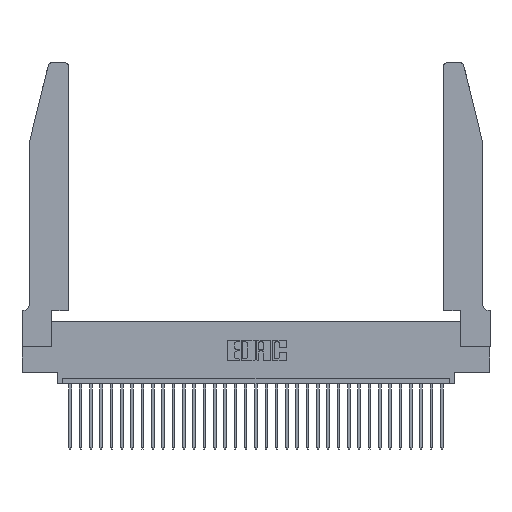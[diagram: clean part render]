
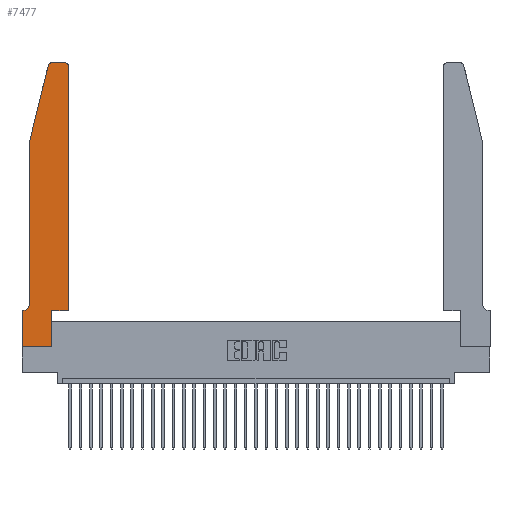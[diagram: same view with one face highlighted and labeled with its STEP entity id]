
A CAD part, top view. The second image highlights one B-rep face of the part: STEP entity #7477.
In plain terms, the highlighted planar face has unit normal (0, 0, 1).
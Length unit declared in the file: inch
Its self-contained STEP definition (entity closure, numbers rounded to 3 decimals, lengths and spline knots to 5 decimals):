
#269 = ORIENTED_EDGE ( 'NONE', *, *, #16460, .T. ) ;
#710 = EDGE_CURVE ( 'NONE', #20700, #3134, #12062, .T. ) ;
#1244 = CARTESIAN_POINT ( 'NONE',  ( 0.2865, 0., 0.37 ) ) ;
#1474 = CARTESIAN_POINT ( 'NONE',  ( 0.2865, 0.35, 0.37 ) ) ;
#1552 = DIRECTION ( 'NONE',  ( 0., 0., 1. ) ) ;
#1914 = ORIENTED_EDGE ( 'NONE', *, *, #18119, .T. ) ;
#2998 = VERTEX_POINT ( 'NONE', #11848 ) ;
#3014 = EDGE_CURVE ( 'NONE', #13553, #13053, #17660, .T. ) ;
#3064 = DIRECTION ( 'NONE',  ( 1., 0., 0. ) ) ;
#3134 = VERTEX_POINT ( 'NONE', #23546 ) ;
#3260 = ORIENTED_EDGE ( 'NONE', *, *, #4579, .T. ) ;
#3296 = EDGE_CURVE ( 'NONE', #10385, #30627, #6318, .T. ) ;
#3411 = CARTESIAN_POINT ( 'NONE',  ( 0.284, 2.72, 0.37 ) ) ;
#4060 = DIRECTION ( 'NONE',  ( -0.239, -0.971, 0. ) ) ;
#4579 = EDGE_CURVE ( 'NONE', #2998, #20700, #14374, .T. ) ;
#4754 = CARTESIAN_POINT ( 'NONE',  ( 0.4205, 2.75, 0.37 ) ) ;
#5296 = CARTESIAN_POINT ( 'NONE',  ( 0.4505, 2.72, 0.37 ) ) ;
#5766 = LINE ( 'NONE', #24744, #9333 ) ;
#6140 = VERTEX_POINT ( 'NONE', #5296 ) ;
#6318 = LINE ( 'NONE', #20263, #19251 ) ;
#6461 = AXIS2_PLACEMENT_3D ( 'NONE', #18483, #29084, #31238 ) ;
#6931 = LINE ( 'NONE', #9393, #11323 ) ;
#7217 = VECTOR ( 'NONE', #20323, 39.37008 ) ;
#7477 = ADVANCED_FACE ( 'NONE', ( #32349 ), #24141, .T. ) ;
#9320 = DIRECTION ( 'NONE',  ( 0., -1., 0. ) ) ;
#9333 = VECTOR ( 'NONE', #27323, 39.37008 ) ;
#9393 = CARTESIAN_POINT ( 'NONE',  ( 0.4505, 0.35, 0.37 ) ) ;
#9917 = EDGE_CURVE ( 'NONE', #13053, #26023, #23790, .T. ) ;
#9991 = CARTESIAN_POINT ( 'NONE',  ( 0.0755, 2., 0.37 ) ) ;
#10385 = VERTEX_POINT ( 'NONE', #25765 ) ;
#11323 = VECTOR ( 'NONE', #17230, 39.37008 ) ;
#11848 = CARTESIAN_POINT ( 'NONE',  ( 0.25487, 2.72718, 0.37 ) ) ;
#12062 = LINE ( 'NONE', #9991, #7217 ) ;
#12169 = AXIS2_PLACEMENT_3D ( 'NONE', #16424, #18497, #3064 ) ;
#12564 = EDGE_CURVE ( 'NONE', #3134, #10385, #16712, .T. ) ;
#12690 = VECTOR ( 'NONE', #17209, 39.37008 ) ;
#13053 = VERTEX_POINT ( 'NONE', #1244 ) ;
#13158 = DIRECTION ( 'NONE',  ( 0., 0., 1. ) ) ;
#13553 = VERTEX_POINT ( 'NONE', #32942 ) ;
#14243 = DIRECTION ( 'NONE',  ( 1., 0., 0. ) ) ;
#14296 = CIRCLE ( 'NONE', #29141, 0.03 ) ;
#14374 = LINE ( 'NONE', #29419, #25291 ) ;
#14668 = DIRECTION ( 'NONE',  ( 1., 0., 0. ) ) ;
#15079 = VERTEX_POINT ( 'NONE', #32220 ) ;
#16300 = LINE ( 'NONE', #19033, #12690 ) ;
#16424 = CARTESIAN_POINT ( 'NONE',  ( 0., 0.35, 0.37 ) ) ;
#16460 = EDGE_CURVE ( 'NONE', #30627, #13553, #33411, .T. ) ;
#16694 = VERTEX_POINT ( 'NONE', #4754 ) ;
#16712 = CIRCLE ( 'NONE', #6461, 0.07 ) ;
#17209 = DIRECTION ( 'NONE',  ( 0., 1., 0. ) ) ;
#17230 = DIRECTION ( 'NONE',  ( 1., 0., 0. ) ) ;
#17652 = CARTESIAN_POINT ( 'NONE',  ( 0.4205, 2.72, 0.37 ) ) ;
#17660 = LINE ( 'NONE', #24529, #19680 ) ;
#18119 = EDGE_CURVE ( 'NONE', #6140, #16694, #14296, .T. ) ;
#18483 = CARTESIAN_POINT ( 'NONE',  ( 0.0055, 0.42, 0.37 ) ) ;
#18497 = DIRECTION ( 'NONE',  ( 0., 0., 1. ) ) ;
#18944 = ORIENTED_EDGE ( 'NONE', *, *, #3014, .T. ) ;
#19033 = CARTESIAN_POINT ( 'NONE',  ( 0.4505, 0.35, 0.37 ) ) ;
#19199 = ORIENTED_EDGE ( 'NONE', *, *, #3296, .T. ) ;
#19251 = VECTOR ( 'NONE', #25452, 39.37008 ) ;
#19324 = CARTESIAN_POINT ( 'NONE',  ( 0.4505, 0.35, 0.37 ) ) ;
#19478 = VERTEX_POINT ( 'NONE', #19324 ) ;
#19511 = DIRECTION ( 'NONE',  ( 0., 1., 0. ) ) ;
#19673 = CARTESIAN_POINT ( 'NONE',  ( 0., 0., 0.37 ) ) ;
#19680 = VECTOR ( 'NONE', #14668, 39.37008 ) ;
#20263 = CARTESIAN_POINT ( 'NONE',  ( 0.0755, 0.35, 0.37 ) ) ;
#20323 = DIRECTION ( 'NONE',  ( 0., -1., 0. ) ) ;
#20700 = VERTEX_POINT ( 'NONE', #21870 ) ;
#20784 = ORIENTED_EDGE ( 'NONE', *, *, #30672, .T. ) ;
#21500 = ORIENTED_EDGE ( 'NONE', *, *, #12564, .T. ) ;
#21706 = CIRCLE ( 'NONE', #27066, 0.03 ) ;
#21870 = CARTESIAN_POINT ( 'NONE',  ( 0.0755, 2., 0.37 ) ) ;
#22115 = VECTOR ( 'NONE', #9320, 39.37008 ) ;
#22261 = ORIENTED_EDGE ( 'NONE', *, *, #24483, .T. ) ;
#22403 = ORIENTED_EDGE ( 'NONE', *, *, #9917, .T. ) ;
#23478 = DIRECTION ( 'NONE',  ( 1., 0., 0. ) ) ;
#23546 = CARTESIAN_POINT ( 'NONE',  ( 0.0755, 0.42, 0.37 ) ) ;
#23790 = LINE ( 'NONE', #1474, #31475 ) ;
#24141 = PLANE ( 'NONE',  #12169 ) ;
#24483 = EDGE_CURVE ( 'NONE', #15079, #2998, #21706, .T. ) ;
#24529 = CARTESIAN_POINT ( 'NONE',  ( 0., 0., 0.37 ) ) ;
#24744 = CARTESIAN_POINT ( 'NONE',  ( 0.2605, 2.75, 0.37 ) ) ;
#25157 = CARTESIAN_POINT ( 'NONE',  ( 0., 0.35, 0.37 ) ) ;
#25291 = VECTOR ( 'NONE', #4060, 39.37008 ) ;
#25452 = DIRECTION ( 'NONE',  ( -1., 0., 0. ) ) ;
#25741 = CARTESIAN_POINT ( 'NONE',  ( 0.2865, 0.35, 0.37 ) ) ;
#25765 = CARTESIAN_POINT ( 'NONE',  ( 0.0055, 0.35, 0.37 ) ) ;
#26023 = VERTEX_POINT ( 'NONE', #25741 ) ;
#27066 = AXIS2_PLACEMENT_3D ( 'NONE', #3411, #13158, #23478 ) ;
#27323 = DIRECTION ( 'NONE',  ( -1., 0., 0. ) ) ;
#29084 = DIRECTION ( 'NONE',  ( 0., 0., -1. ) ) ;
#29141 = AXIS2_PLACEMENT_3D ( 'NONE', #17652, #1552, #14243 ) ;
#29255 = ORIENTED_EDGE ( 'NONE', *, *, #32488, .T. ) ;
#29419 = CARTESIAN_POINT ( 'NONE',  ( 0.0755, 2., 0.37 ) ) ;
#29527 = EDGE_LOOP ( 'NONE', ( #30228, #22261, #3260, #31024, #21500, #19199, #269, #18944, #22403, #29255, #20784, #1914 ) ) ;
#30228 = ORIENTED_EDGE ( 'NONE', *, *, #31842, .T. ) ;
#30627 = VERTEX_POINT ( 'NONE', #25157 ) ;
#30672 = EDGE_CURVE ( 'NONE', #19478, #6140, #16300, .T. ) ;
#31024 = ORIENTED_EDGE ( 'NONE', *, *, #710, .T. ) ;
#31238 = DIRECTION ( 'NONE',  ( -1., 0., 0. ) ) ;
#31475 = VECTOR ( 'NONE', #19511, 39.37008 ) ;
#31842 = EDGE_CURVE ( 'NONE', #16694, #15079, #5766, .T. ) ;
#32220 = CARTESIAN_POINT ( 'NONE',  ( 0.284, 2.75, 0.37 ) ) ;
#32349 = FACE_OUTER_BOUND ( 'NONE', #29527, .T. ) ;
#32488 = EDGE_CURVE ( 'NONE', #26023, #19478, #6931, .T. ) ;
#32942 = CARTESIAN_POINT ( 'NONE',  ( 0., 0., 0.37 ) ) ;
#33411 = LINE ( 'NONE', #19673, #22115 ) ;
